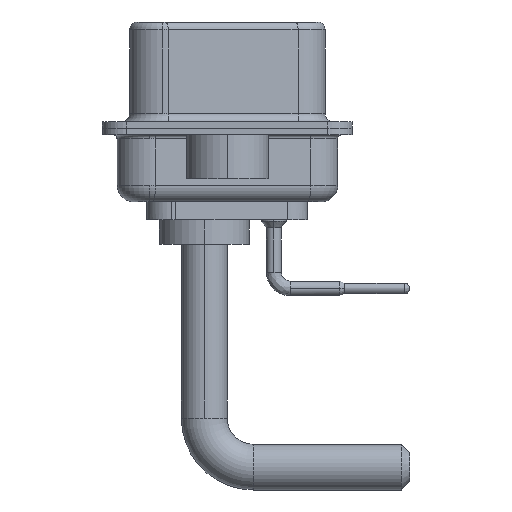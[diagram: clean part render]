
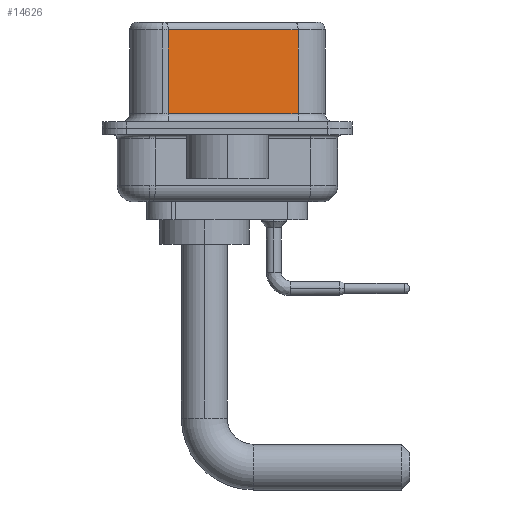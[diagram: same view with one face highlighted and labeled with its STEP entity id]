
A CAD part, left-side view. The second image highlights one B-rep face of the part: STEP entity #14626.
In plain terms, the highlighted planar face has unit normal (-0.985, -0.174, 0).
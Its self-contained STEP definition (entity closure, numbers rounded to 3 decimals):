
#871 = PLANE ( 'NONE',  #5065 ) ;
#2302 = CARTESIAN_POINT ( 'NONE',  ( 5.132, -4.322, 6.02 ) ) ;
#3628 = VECTOR ( 'NONE', #7444, 1000. ) ;
#4846 = ORIENTED_EDGE ( 'NONE', *, *, #6337, .T. ) ;
#4867 = EDGE_LOOP ( 'NONE', ( #19258, #4846, #18526, #12323 ) ) ;
#5065 = AXIS2_PLACEMENT_3D ( 'NONE', #8245, #6439, #13840 ) ;
#5452 = VERTEX_POINT ( 'NONE', #11349 ) ;
#6337 = EDGE_CURVE ( 'NONE', #20542, #5452, #8978, .T. ) ;
#6439 = DIRECTION ( 'NONE',  ( 0.985, 0.174, 0. ) ) ;
#7444 = DIRECTION ( 'NONE',  ( 0.174, -0.985, 0. ) ) ;
#8072 = VERTEX_POINT ( 'NONE', #14230 ) ;
#8245 = CARTESIAN_POINT ( 'NONE',  ( 5.132, -4.322, 6.52 ) ) ;
#8632 = EDGE_CURVE ( 'NONE', #20542, #19171, #18181, .T. ) ;
#8978 = LINE ( 'NONE', #23862, #21861 ) ;
#10725 = VECTOR ( 'NONE', #11015, 1000. ) ;
#10913 = LINE ( 'NONE', #14690, #22886 ) ;
#11015 = DIRECTION ( 'NONE',  ( 0., 0., -1. ) ) ;
#11349 = CARTESIAN_POINT ( 'NONE',  ( 3.73, 3.628, 6.02 ) ) ;
#12323 = ORIENTED_EDGE ( 'NONE', *, *, #19409, .T. ) ;
#12396 = DIRECTION ( 'NONE',  ( 0., 0., -1. ) ) ;
#12567 = LINE ( 'NONE', #20284, #3628 ) ;
#13111 = DIRECTION ( 'NONE',  ( -0.174, 0.985, 0. ) ) ;
#13531 = CARTESIAN_POINT ( 'NONE',  ( 5.132, -4.322, 0.9 ) ) ;
#13840 = DIRECTION ( 'NONE',  ( -0.174, 0.985, 0. ) ) ;
#14230 = CARTESIAN_POINT ( 'NONE',  ( 3.73, 3.628, 0.9 ) ) ;
#14626 = ADVANCED_FACE ( 'NONE', ( #17464 ), #871, .F. ) ;
#14690 = CARTESIAN_POINT ( 'NONE',  ( 3.73, 3.628, 6.52 ) ) ;
#16848 = CARTESIAN_POINT ( 'NONE',  ( 5.132, -4.322, 6.52 ) ) ;
#17464 = FACE_OUTER_BOUND ( 'NONE', #4867, .T. ) ;
#17689 = EDGE_CURVE ( 'NONE', #5452, #8072, #10913, .T. ) ;
#18181 = LINE ( 'NONE', #16848, #10725 ) ;
#18526 = ORIENTED_EDGE ( 'NONE', *, *, #17689, .T. ) ;
#19171 = VERTEX_POINT ( 'NONE', #13531 ) ;
#19258 = ORIENTED_EDGE ( 'NONE', *, *, #8632, .F. ) ;
#19409 = EDGE_CURVE ( 'NONE', #8072, #19171, #12567, .T. ) ;
#20284 = CARTESIAN_POINT ( 'NONE',  ( 5.132, -4.322, 0.9 ) ) ;
#20542 = VERTEX_POINT ( 'NONE', #2302 ) ;
#21861 = VECTOR ( 'NONE', #13111, 1000. ) ;
#22886 = VECTOR ( 'NONE', #12396, 1000. ) ;
#23862 = CARTESIAN_POINT ( 'NONE',  ( 5.132, -4.322, 6.02 ) ) ;
